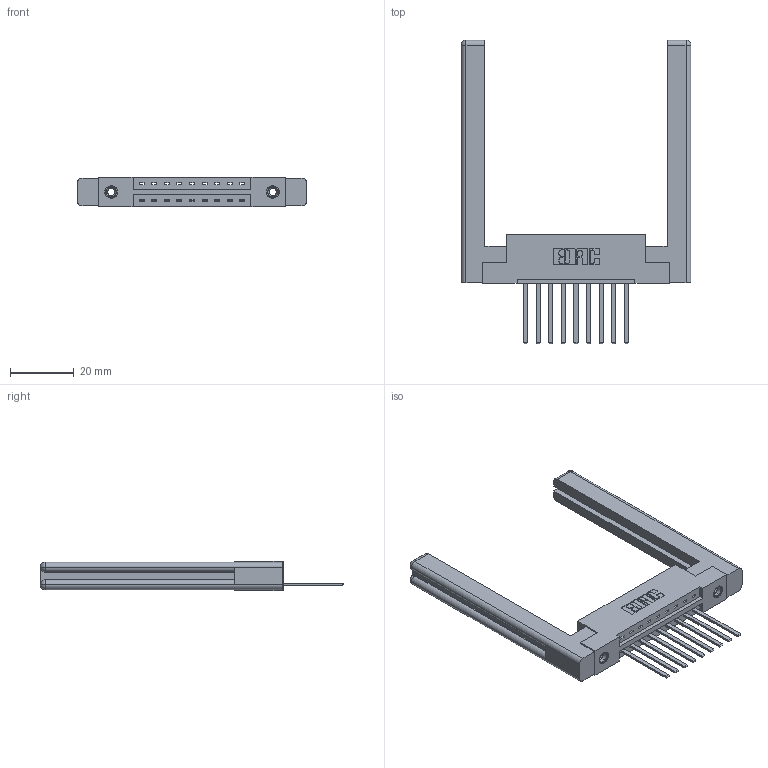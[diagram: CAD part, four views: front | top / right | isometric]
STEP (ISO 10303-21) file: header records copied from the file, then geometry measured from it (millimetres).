
FILE_DESCRIPTION (( 'STEP AP203' ), '1' );
FILE_NAME ('387-009-544-158.STEP', '2019-10-02T10:49:29', ( '' ), ( '' ), 'SwSTEP 2.0', 'SolidWorks 2016', '' );
FILE_SCHEMA (( 'CONFIG_CONTROL_DESIGN' ));
Length unit declared in the file: inch
Products named in the file (5): 345-292-001_345-293-144; 387-009-544-158; 337 Part_Flush Mounting Lugs - 0.156 Dia-TI; 307-220-058; 345-250-001_345-250-001-102
Assembly tree (14 placements, depth 2):
  387-009-544-158
    337 Part_Flush Mounting Lugs - 0.156 Dia-TI
    345-292-001_345-293-144  x9
    345-250-001_345-250-001-102  x2
    307-220-058  x2
Bounding box: 72.29 x 95.38 x 9.4 mm (x, y, z)
Volume: 14366.6 mm3; surface area: 12817.5 mm2
Topology: 14 solids, 14 shells, 760 faces, 2195 edges, 1438 vertices
Faces by surface type: plane 532, cylinder 204, cone 12, torus 12
Entity records: 13408 total; most frequent: CARTESIAN_POINT 2332, ORIENTED_EDGE 2216, DIRECTION 2046, EDGE_CURVE 1108, LINE 936, VECTOR 936, VERTEX_POINT 730, AXIS2_PLACEMENT_3D 555
